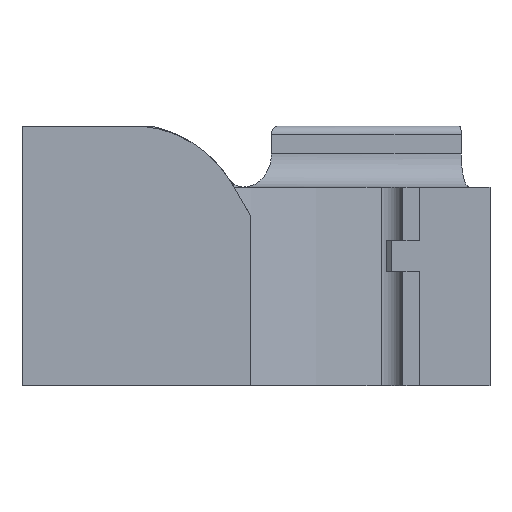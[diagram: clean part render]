
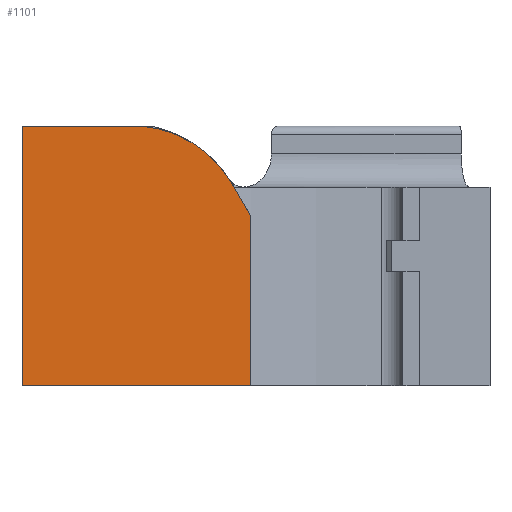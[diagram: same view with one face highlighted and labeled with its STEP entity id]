
A CAD part, front view. The second image highlights one B-rep face of the part: STEP entity #1101.
In plain terms, the highlighted planar face has unit normal (0, -1, 0).
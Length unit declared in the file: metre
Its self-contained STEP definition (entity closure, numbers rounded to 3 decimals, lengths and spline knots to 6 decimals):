
#40=PLANE('',#1227);
#86=FACE_OUTER_BOUND('',#144,.T.);
#144=EDGE_LOOP('',(#925,#926,#927,#928,#929,#930));
#186=LINE('',#1602,#297);
#195=LINE('',#1626,#306);
#213=LINE('',#1678,#324);
#231=LINE('',#1752,#342);
#236=LINE('',#1769,#347);
#297=VECTOR('',#1267,0.01);
#306=VECTOR('',#1288,0.01);
#324=VECTOR('',#1334,0.016179);
#342=VECTOR('',#1396,0.014606);
#347=VECTOR('',#1411,0.01);
#407=CIRCLE('',#1154,0.005582);
#448=VERTEX_POINT('',#1599);
#449=VERTEX_POINT('',#1601);
#451=VERTEX_POINT('',#1607);
#458=VERTEX_POINT('',#1625);
#478=VERTEX_POINT('',#1677);
#512=VERTEX_POINT('',#1750);
#557=EDGE_CURVE('',#449,#448,#186,.T.);
#561=EDGE_CURVE('',#448,#451,#407,.T.);
#569=EDGE_CURVE('',#458,#449,#195,.T.);
#595=EDGE_CURVE('',#478,#458,#213,.T.);
#633=EDGE_CURVE('',#512,#451,#231,.T.);
#640=EDGE_CURVE('',#512,#478,#236,.T.);
#925=ORIENTED_EDGE('',*,*,#640,.T.);
#926=ORIENTED_EDGE('',*,*,#595,.T.);
#927=ORIENTED_EDGE('',*,*,#569,.T.);
#928=ORIENTED_EDGE('',*,*,#557,.T.);
#929=ORIENTED_EDGE('',*,*,#561,.T.);
#930=ORIENTED_EDGE('',*,*,#633,.F.);
#1101=ADVANCED_FACE('',(#86),#40,.F.);
#1154=AXIS2_PLACEMENT_3D('',#1609,#1274,#1275);
#1227=AXIS2_PLACEMENT_3D('',#1893,#1505,#1506);
#1267=DIRECTION('',(-0.505,0.,0.863));
#1274=DIRECTION('center_axis',(0.,-1.,0.));
#1275=DIRECTION('ref_axis',(0.844,0.,0.536));
#1288=DIRECTION('',(0.,0.,1.));
#1334=DIRECTION('',(1.,0.,0.));
#1396=DIRECTION('',(1.,0.,0.));
#1411=DIRECTION('',(0.,0.,-1.));
#1505=DIRECTION('center_axis',(0.,1.,0.));
#1506=DIRECTION('ref_axis',(-1.,0.,0.));
#1599=CARTESIAN_POINT('',(0.014302,-0.00635,0.003058));
#1601=CARTESIAN_POINT('',(0.015312,-0.00635,0.00133));
#1602=CARTESIAN_POINT('',(0.014512,-0.00635,0.002699));
#1607=CARTESIAN_POINT('',(0.010128,-0.00635,0.00562));
#1609=CARTESIAN_POINT('Origin',(0.009592,-0.00635,0.000064));
#1625=CARTESIAN_POINT('',(0.015312,-0.00635,-0.006826));
#1626=CARTESIAN_POINT('',(0.015312,-0.00635,-0.006826));
#1677=CARTESIAN_POINT('',(0.004366,-0.00635,-0.006826));
#1678=CARTESIAN_POINT('',(-0.00605,-0.00635,-0.006826));
#1750=CARTESIAN_POINT('',(0.004366,-0.00635,0.00562));
#1752=CARTESIAN_POINT('',(-0.00605,-0.00635,0.00562));
#1769=CARTESIAN_POINT('',(0.004366,-0.00635,0.00562));
#1893=CARTESIAN_POINT('Origin',(-0.000603,-0.00635,0.00562));
